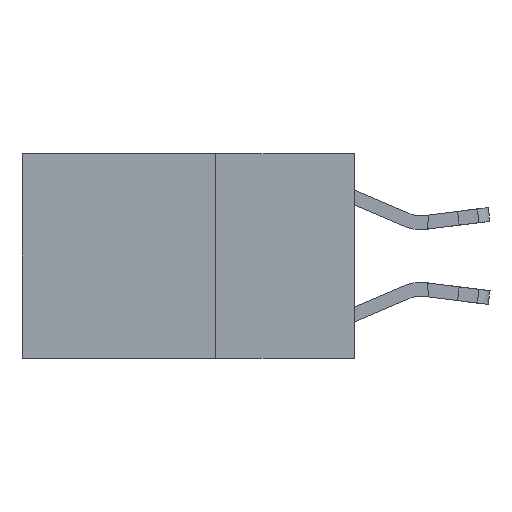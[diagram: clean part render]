
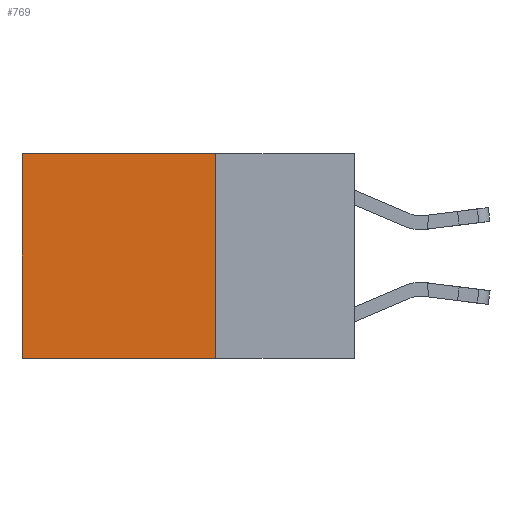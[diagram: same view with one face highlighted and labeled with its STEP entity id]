
A CAD part, left-side view. The second image highlights one B-rep face of the part: STEP entity #769.
In plain terms, the highlighted planar face has unit normal (-1, 0, 0).
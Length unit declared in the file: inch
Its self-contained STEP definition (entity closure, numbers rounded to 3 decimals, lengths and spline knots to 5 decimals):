
#312 = CARTESIAN_POINT ( 'NONE',  ( 0.2625, 0.25, 0. ) ) ;
#769 = ADVANCED_FACE ( 'NONE', ( #8545 ), #2633, .F. ) ;
#946 = CARTESIAN_POINT ( 'NONE',  ( 0.2625, 0.25, -0.37 ) ) ;
#1873 = VERTEX_POINT ( 'NONE', #11020 ) ;
#2633 = PLANE ( 'NONE',  #6980 ) ;
#2650 = EDGE_CURVE ( 'NONE', #9337, #1873, #5472, .T. ) ;
#2914 = EDGE_CURVE ( 'NONE', #10817, #12304, #9784, .T. ) ;
#3085 = EDGE_LOOP ( 'NONE', ( #6686, #9358, #12326, #7308 ) ) ;
#3205 = VECTOR ( 'NONE', #3379, 39.37008 ) ;
#3379 = DIRECTION ( 'NONE',  ( 0., 0., -1. ) ) ;
#3644 = DIRECTION ( 'NONE',  ( 0., 0., -1. ) ) ;
#3859 = LINE ( 'NONE', #11500, #3205 ) ;
#4352 = EDGE_CURVE ( 'NONE', #12304, #1873, #3859, .T. ) ;
#4364 = DIRECTION ( 'NONE',  ( 0., 0., -1. ) ) ;
#5472 = LINE ( 'NONE', #946, #13157 ) ;
#5574 = CARTESIAN_POINT ( 'NONE',  ( 0.2625, 0.25, -0.37 ) ) ;
#6170 = LINE ( 'NONE', #8426, #6499 ) ;
#6499 = VECTOR ( 'NONE', #4364, 39.37008 ) ;
#6515 = DIRECTION ( 'NONE',  ( 0., 1., 0. ) ) ;
#6686 = ORIENTED_EDGE ( 'NONE', *, *, #4352, .T. ) ;
#6980 = AXIS2_PLACEMENT_3D ( 'NONE', #312, #9743, #3644 ) ;
#7308 = ORIENTED_EDGE ( 'NONE', *, *, #2914, .T. ) ;
#8240 = DIRECTION ( 'NONE',  ( 0., 1., 0. ) ) ;
#8426 = CARTESIAN_POINT ( 'NONE',  ( 0.2625, 0.25, 0. ) ) ;
#8545 = FACE_OUTER_BOUND ( 'NONE', #3085, .T. ) ;
#8710 = CARTESIAN_POINT ( 'NONE',  ( 0.2625, 0.6, 0. ) ) ;
#8748 = CARTESIAN_POINT ( 'NONE',  ( 0.2625, 0.25, 0. ) ) ;
#9165 = EDGE_CURVE ( 'NONE', #10817, #9337, #6170, .T. ) ;
#9337 = VERTEX_POINT ( 'NONE', #5574 ) ;
#9358 = ORIENTED_EDGE ( 'NONE', *, *, #2650, .F. ) ;
#9743 = DIRECTION ( 'NONE',  ( 1., 0., 0. ) ) ;
#9784 = LINE ( 'NONE', #11527, #12121 ) ;
#10817 = VERTEX_POINT ( 'NONE', #8748 ) ;
#11020 = CARTESIAN_POINT ( 'NONE',  ( 0.2625, 0.6, -0.37 ) ) ;
#11500 = CARTESIAN_POINT ( 'NONE',  ( 0.2625, 0.6, 0. ) ) ;
#11527 = CARTESIAN_POINT ( 'NONE',  ( 0.2625, 0.25, 0. ) ) ;
#12121 = VECTOR ( 'NONE', #6515, 39.37008 ) ;
#12304 = VERTEX_POINT ( 'NONE', #8710 ) ;
#12326 = ORIENTED_EDGE ( 'NONE', *, *, #9165, .F. ) ;
#13157 = VECTOR ( 'NONE', #8240, 39.37008 ) ;
